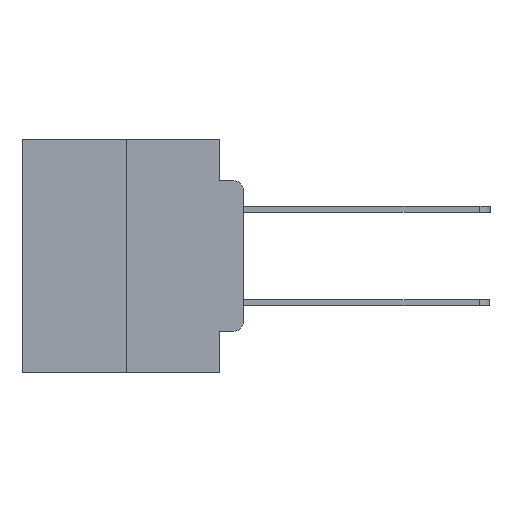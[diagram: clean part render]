
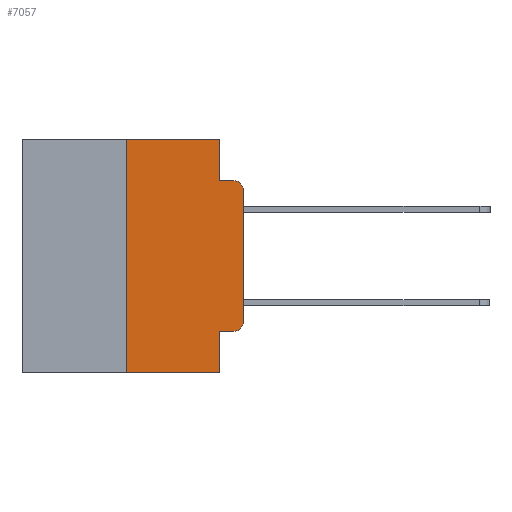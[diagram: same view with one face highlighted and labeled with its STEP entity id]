
A CAD part, left-side view. The second image highlights one B-rep face of the part: STEP entity #7057.
In plain terms, the highlighted planar face has unit normal (-1, 0, 0).
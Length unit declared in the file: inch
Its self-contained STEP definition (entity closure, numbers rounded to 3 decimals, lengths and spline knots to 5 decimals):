
#101 = CARTESIAN_POINT ( 'NONE',  ( 0., 0.473, 0. ) ) ;
#303 = CARTESIAN_POINT ( 'NONE',  ( 0., 0., -0.1085 ) ) ;
#493 = ORIENTED_EDGE ( 'NONE', *, *, #17911, .T. ) ;
#1051 = EDGE_CURVE ( 'NONE', #26050, #15069, #23920, .T. ) ;
#1535 = DIRECTION ( 'NONE',  ( -1., 0., 0. ) ) ;
#1599 = LINE ( 'NONE', #7473, #18773 ) ;
#1727 = CARTESIAN_POINT ( 'NONE',  ( 0., 0.25, 0. ) ) ;
#1926 = VERTEX_POINT ( 'NONE', #15609 ) ;
#2452 = VERTEX_POINT ( 'NONE', #10593 ) ;
#3413 = CARTESIAN_POINT ( 'NONE',  ( 0., 0., 0. ) ) ;
#3624 = CARTESIAN_POINT ( 'NONE',  ( 0., 0.051, -0.5 ) ) ;
#3799 = CIRCLE ( 'NONE', #26143, 0.02 ) ;
#4178 = EDGE_CURVE ( 'NONE', #7048, #10024, #3799, .T. ) ;
#4319 = VECTOR ( 'NONE', #23950, 39.37008 ) ;
#4372 = LINE ( 'NONE', #3413, #21792 ) ;
#4686 = VERTEX_POINT ( 'NONE', #5351 ) ;
#5004 = LINE ( 'NONE', #27696, #4319 ) ;
#5351 = CARTESIAN_POINT ( 'NONE',  ( 0., 0.051, 0. ) ) ;
#5904 = CARTESIAN_POINT ( 'NONE',  ( 0., 0.051, -0.4115 ) ) ;
#5995 = LINE ( 'NONE', #9934, #22718 ) ;
#6401 = VECTOR ( 'NONE', #11206, 39.37008 ) ;
#6558 = EDGE_CURVE ( 'NONE', #1926, #10024, #1599, .T. ) ;
#7048 = VERTEX_POINT ( 'NONE', #303 ) ;
#7057 = ADVANCED_FACE ( 'NONE', ( #23127 ), #22199, .F. ) ;
#7473 = CARTESIAN_POINT ( 'NONE',  ( 0., 0.051, -0.0885 ) ) ;
#8040 = EDGE_CURVE ( 'NONE', #19943, #22096, #5004, .T. ) ;
#8462 = CARTESIAN_POINT ( 'NONE',  ( 0., 0.051, -0.4115 ) ) ;
#9140 = CARTESIAN_POINT ( 'NONE',  ( 0., 0.473, 0. ) ) ;
#9152 = ORIENTED_EDGE ( 'NONE', *, *, #20113, .F. ) ;
#9382 = CARTESIAN_POINT ( 'NONE',  ( 0., 0.25, -0.5 ) ) ;
#9647 = DIRECTION ( 'NONE',  ( 0., -1., 0. ) ) ;
#9934 = CARTESIAN_POINT ( 'NONE',  ( 0., 0.051, 0. ) ) ;
#10005 = DIRECTION ( 'NONE',  ( 0., -1., 0. ) ) ;
#10024 = VERTEX_POINT ( 'NONE', #23946 ) ;
#10314 = ORIENTED_EDGE ( 'NONE', *, *, #18302, .F. ) ;
#10593 = CARTESIAN_POINT ( 'NONE',  ( 0., 0., -0.3915 ) ) ;
#10640 = CARTESIAN_POINT ( 'NONE',  ( 0., 0.02, -0.3915 ) ) ;
#10643 = ORIENTED_EDGE ( 'NONE', *, *, #6558, .F. ) ;
#11206 = DIRECTION ( 'NONE',  ( 0., 0., -1. ) ) ;
#11308 = DIRECTION ( 'NONE',  ( 0., 0., -1. ) ) ;
#11948 = ORIENTED_EDGE ( 'NONE', *, *, #16428, .F. ) ;
#12211 = LINE ( 'NONE', #19922, #6401 ) ;
#12669 = ORIENTED_EDGE ( 'NONE', *, *, #4178, .T. ) ;
#12861 = DIRECTION ( 'NONE',  ( 0., 0., -1. ) ) ;
#13737 = VECTOR ( 'NONE', #10005, 39.37008 ) ;
#14139 = VECTOR ( 'NONE', #14944, 39.37008 ) ;
#14656 = CARTESIAN_POINT ( 'NONE',  ( 0., 0.02, -0.1085 ) ) ;
#14944 = DIRECTION ( 'NONE',  ( 0., 0., 1. ) ) ;
#15069 = VERTEX_POINT ( 'NONE', #15148 ) ;
#15148 = CARTESIAN_POINT ( 'NONE',  ( 0., 0.02, -0.4115 ) ) ;
#15455 = DIRECTION ( 'NONE',  ( 0., -1., 0. ) ) ;
#15609 = CARTESIAN_POINT ( 'NONE',  ( 0., 0.051, -0.0885 ) ) ;
#16428 = EDGE_CURVE ( 'NONE', #26592, #4686, #25227, .T. ) ;
#16464 = AXIS2_PLACEMENT_3D ( 'NONE', #9140, #24371, #11308 ) ;
#16854 = DIRECTION ( 'NONE',  ( 0., 0., -1. ) ) ;
#16873 = ORIENTED_EDGE ( 'NONE', *, *, #1051, .T. ) ;
#17739 = AXIS2_PLACEMENT_3D ( 'NONE', #10640, #25827, #12861 ) ;
#17911 = EDGE_CURVE ( 'NONE', #2452, #7048, #4372, .T. ) ;
#18302 = EDGE_CURVE ( 'NONE', #4686, #1926, #12211, .T. ) ;
#18651 = DIRECTION ( 'NONE',  ( 0., 0., -1. ) ) ;
#18773 = VECTOR ( 'NONE', #9647, 39.37008 ) ;
#19508 = VECTOR ( 'NONE', #15455, 39.37008 ) ;
#19922 = CARTESIAN_POINT ( 'NONE',  ( 0., 0.051, 0. ) ) ;
#19943 = VERTEX_POINT ( 'NONE', #9382 ) ;
#20113 = EDGE_CURVE ( 'NONE', #26050, #22096, #5995, .T. ) ;
#20624 = EDGE_LOOP ( 'NONE', ( #493, #12669, #10643, #10314, #11948, #21515, #25969, #9152, #16873, #25913 ) ) ;
#21515 = ORIENTED_EDGE ( 'NONE', *, *, #21579, .F. ) ;
#21579 = EDGE_CURVE ( 'NONE', #19943, #26592, #25622, .T. ) ;
#21792 = VECTOR ( 'NONE', #22968, 39.37008 ) ;
#22096 = VERTEX_POINT ( 'NONE', #3624 ) ;
#22199 = PLANE ( 'NONE',  #16464 ) ;
#22718 = VECTOR ( 'NONE', #18651, 39.37008 ) ;
#22968 = DIRECTION ( 'NONE',  ( 0., 0., 1. ) ) ;
#23127 = FACE_OUTER_BOUND ( 'NONE', #20624, .T. ) ;
#23856 = CARTESIAN_POINT ( 'NONE',  ( 0., 0.25, 0. ) ) ;
#23920 = LINE ( 'NONE', #5904, #13737 ) ;
#23946 = CARTESIAN_POINT ( 'NONE',  ( 0., 0.02, -0.0885 ) ) ;
#23950 = DIRECTION ( 'NONE',  ( 0., -1., 0. ) ) ;
#24371 = DIRECTION ( 'NONE',  ( 1., 0., 0. ) ) ;
#25227 = LINE ( 'NONE', #101, #19508 ) ;
#25622 = LINE ( 'NONE', #1727, #14139 ) ;
#25827 = DIRECTION ( 'NONE',  ( -1., 0., 0. ) ) ;
#25913 = ORIENTED_EDGE ( 'NONE', *, *, #27769, .T. ) ;
#25969 = ORIENTED_EDGE ( 'NONE', *, *, #8040, .T. ) ;
#26050 = VERTEX_POINT ( 'NONE', #8462 ) ;
#26143 = AXIS2_PLACEMENT_3D ( 'NONE', #14656, #1535, #16854 ) ;
#26592 = VERTEX_POINT ( 'NONE', #23856 ) ;
#27314 = CIRCLE ( 'NONE', #17739, 0.02 ) ;
#27696 = CARTESIAN_POINT ( 'NONE',  ( 0., 0.473, -0.5 ) ) ;
#27769 = EDGE_CURVE ( 'NONE', #15069, #2452, #27314, .T. ) ;
